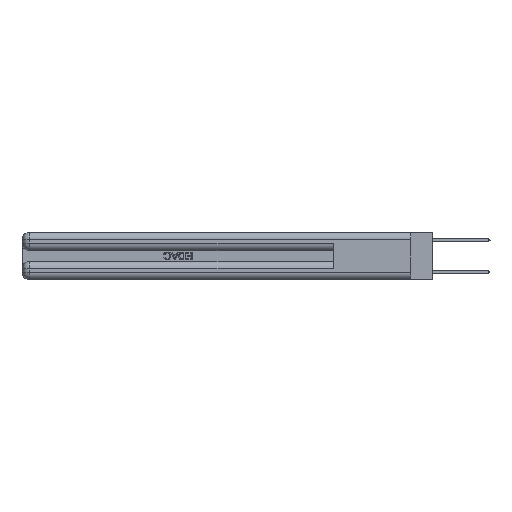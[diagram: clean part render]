
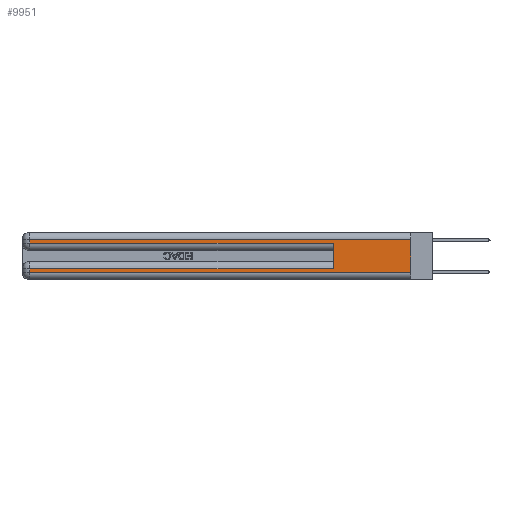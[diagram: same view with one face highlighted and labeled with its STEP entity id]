
A CAD part, left-side view. The second image highlights one B-rep face of the part: STEP entity #9951.
In plain terms, the highlighted planar face has unit normal (-1, 0, 0).
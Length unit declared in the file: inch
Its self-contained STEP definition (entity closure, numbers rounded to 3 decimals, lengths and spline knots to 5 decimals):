
#223 = VERTEX_POINT ( 'NONE', #28321 ) ;
#327 = VECTOR ( 'NONE', #15754, 39.37008 ) ;
#543 = CARTESIAN_POINT ( 'NONE',  ( 0., 0.6, 0.145 ) ) ;
#661 = ORIENTED_EDGE ( 'NONE', *, *, #15108, .T. ) ;
#1140 = VERTEX_POINT ( 'NONE', #29237 ) ;
#2374 = VERTEX_POINT ( 'NONE', #19567 ) ;
#3146 = VECTOR ( 'NONE', #14184, 39.37008 ) ;
#3993 = CARTESIAN_POINT ( 'NONE',  ( 0., 2.94, 0.06 ) ) ;
#4411 = VERTEX_POINT ( 'NONE', #8236 ) ;
#4414 = DIRECTION ( 'NONE',  ( 0., 1., 0. ) ) ;
#4659 = LINE ( 'NONE', #5916, #23265 ) ;
#4873 = EDGE_CURVE ( 'NONE', #7147, #19104, #15142, .T. ) ;
#5336 = VECTOR ( 'NONE', #26522, 39.37008 ) ;
#5714 = EDGE_LOOP ( 'NONE', ( #30346, #11031, #17768, #5844, #19332, #661, #7435, #28408 ) ) ;
#5844 = ORIENTED_EDGE ( 'NONE', *, *, #28608, .T. ) ;
#5916 = CARTESIAN_POINT ( 'NONE',  ( 0., 0., 0.37 ) ) ;
#7051 = VECTOR ( 'NONE', #30854, 39.37008 ) ;
#7147 = VERTEX_POINT ( 'NONE', #15452 ) ;
#7435 = ORIENTED_EDGE ( 'NONE', *, *, #4873, .T. ) ;
#7640 = EDGE_CURVE ( 'NONE', #223, #1140, #23209, .T. ) ;
#8090 = FACE_OUTER_BOUND ( 'NONE', #5714, .T. ) ;
#8236 = CARTESIAN_POINT ( 'NONE',  ( 0., 0., 0.06 ) ) ;
#9807 = VECTOR ( 'NONE', #4414, 39.37008 ) ;
#9934 = CARTESIAN_POINT ( 'NONE',  ( 0., 2.94, 0.285 ) ) ;
#9938 = LINE ( 'NONE', #26750, #3146 ) ;
#9951 = ADVANCED_FACE ( 'NONE', ( #8090 ), #29274, .F. ) ;
#10816 = LINE ( 'NONE', #14660, #30156 ) ;
#11031 = ORIENTED_EDGE ( 'NONE', *, *, #7640, .T. ) ;
#11538 = CARTESIAN_POINT ( 'NONE',  ( 0., 0., 0.37 ) ) ;
#13551 = VECTOR ( 'NONE', #20177, 39.37008 ) ;
#13949 = CARTESIAN_POINT ( 'NONE',  ( 0., 0., 0.285 ) ) ;
#14184 = DIRECTION ( 'NONE',  ( 0., -1., 0. ) ) ;
#14239 = VERTEX_POINT ( 'NONE', #9934 ) ;
#14409 = CARTESIAN_POINT ( 'NONE',  ( 0., 0.6, 0.285 ) ) ;
#14660 = CARTESIAN_POINT ( 'NONE',  ( 0., 2.94, 0.37 ) ) ;
#15108 = EDGE_CURVE ( 'NONE', #2374, #7147, #20595, .T. ) ;
#15142 = LINE ( 'NONE', #17651, #13551 ) ;
#15452 = CARTESIAN_POINT ( 'NONE',  ( 0., 2.94, 0.085 ) ) ;
#15754 = DIRECTION ( 'NONE',  ( 0., 1., 0. ) ) ;
#15786 = VERTEX_POINT ( 'NONE', #14409 ) ;
#16047 = DIRECTION ( 'NONE',  ( 0., 0., -1. ) ) ;
#16175 = EDGE_CURVE ( 'NONE', #223, #4411, #4659, .T. ) ;
#16720 = DIRECTION ( 'NONE',  ( 0., 0., -1. ) ) ;
#16790 = EDGE_CURVE ( 'NONE', #2374, #15786, #20536, .T. ) ;
#17651 = CARTESIAN_POINT ( 'NONE',  ( 0., 2.94, 0.37 ) ) ;
#17768 = ORIENTED_EDGE ( 'NONE', *, *, #30279, .T. ) ;
#19104 = VERTEX_POINT ( 'NONE', #3993 ) ;
#19332 = ORIENTED_EDGE ( 'NONE', *, *, #16790, .F. ) ;
#19567 = CARTESIAN_POINT ( 'NONE',  ( 0., 0.6, 0.085 ) ) ;
#20177 = DIRECTION ( 'NONE',  ( 0., 0., -1. ) ) ;
#20536 = LINE ( 'NONE', #543, #7051 ) ;
#20595 = LINE ( 'NONE', #28309, #327 ) ;
#23209 = LINE ( 'NONE', #29740, #9807 ) ;
#23265 = VECTOR ( 'NONE', #16047, 39.37008 ) ;
#24225 = AXIS2_PLACEMENT_3D ( 'NONE', #11538, #31790, #16720 ) ;
#25545 = LINE ( 'NONE', #13949, #5336 ) ;
#25863 = EDGE_CURVE ( 'NONE', #19104, #4411, #9938, .T. ) ;
#26522 = DIRECTION ( 'NONE',  ( 0., -1., 0. ) ) ;
#26750 = CARTESIAN_POINT ( 'NONE',  ( 0., 0., 0.06 ) ) ;
#28309 = CARTESIAN_POINT ( 'NONE',  ( 0., 0., 0.085 ) ) ;
#28321 = CARTESIAN_POINT ( 'NONE',  ( 0., 0., 0.31 ) ) ;
#28408 = ORIENTED_EDGE ( 'NONE', *, *, #25863, .T. ) ;
#28608 = EDGE_CURVE ( 'NONE', #14239, #15786, #25545, .T. ) ;
#29237 = CARTESIAN_POINT ( 'NONE',  ( 0., 2.94, 0.31 ) ) ;
#29274 = PLANE ( 'NONE',  #24225 ) ;
#29740 = CARTESIAN_POINT ( 'NONE',  ( 0., 0., 0.31 ) ) ;
#30156 = VECTOR ( 'NONE', #32266, 39.37008 ) ;
#30279 = EDGE_CURVE ( 'NONE', #1140, #14239, #10816, .T. ) ;
#30346 = ORIENTED_EDGE ( 'NONE', *, *, #16175, .F. ) ;
#30854 = DIRECTION ( 'NONE',  ( 0., 0., 1. ) ) ;
#31790 = DIRECTION ( 'NONE',  ( 1., 0., 0. ) ) ;
#32266 = DIRECTION ( 'NONE',  ( 0., 0., -1. ) ) ;
